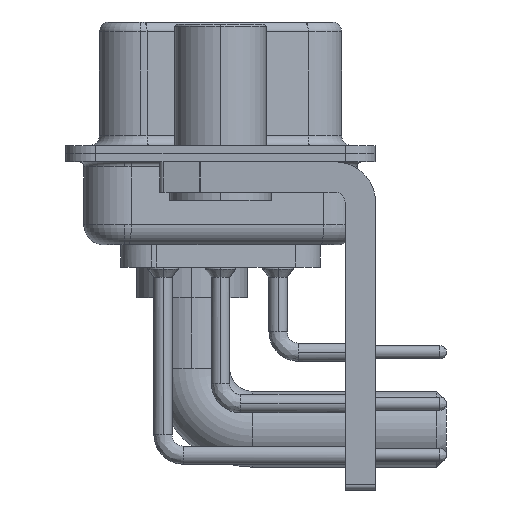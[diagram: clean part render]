
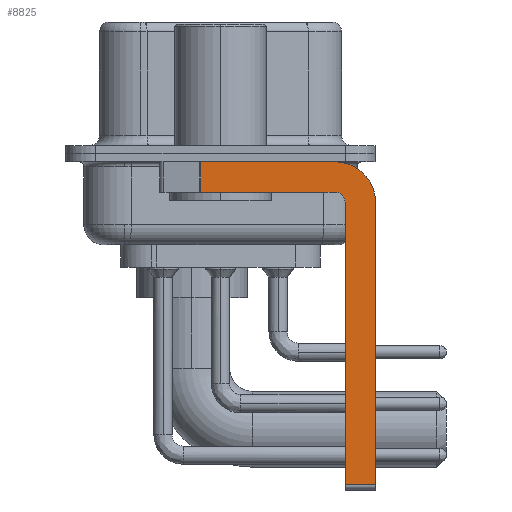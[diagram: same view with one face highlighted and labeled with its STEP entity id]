
A CAD part, left-side view. The second image highlights one B-rep face of the part: STEP entity #8825.
In plain terms, the highlighted planar face has unit normal (-1, 0, 0).
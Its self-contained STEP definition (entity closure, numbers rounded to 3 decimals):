
#295 = EDGE_LOOP ( 'NONE', ( #24912, #34311, #26086, #13538, #4832, #24836, #29060, #19026 ) ) ;
#925 = EDGE_CURVE ( 'NONE', #3163, #36008, #24729, .T. ) ;
#1463 = LINE ( 'NONE', #37172, #24164 ) ;
#2864 = VERTEX_POINT ( 'NONE', #9417 ) ;
#3163 = VERTEX_POINT ( 'NONE', #17668 ) ;
#3629 = CARTESIAN_POINT ( 'NONE',  ( -2.9, -5.65, -2.4 ) ) ;
#4257 = CIRCLE ( 'NONE', #36203, 2. ) ;
#4462 = VERTEX_POINT ( 'NONE', #5846 ) ;
#4832 = ORIENTED_EDGE ( 'NONE', *, *, #34094, .F. ) ;
#5170 = CARTESIAN_POINT ( 'NONE',  ( -2.9, -5.65, -2.4 ) ) ;
#5846 = CARTESIAN_POINT ( 'NONE',  ( -2.9, -5.65, -1.9 ) ) ;
#6271 = CARTESIAN_POINT ( 'NONE',  ( -2.9, -6.15, -16.6 ) ) ;
#6562 = DIRECTION ( 'NONE',  ( 0., -1., 0. ) ) ;
#7329 = EDGE_CURVE ( 'NONE', #3163, #32283, #21531, .T. ) ;
#7359 = DIRECTION ( 'NONE',  ( 0., 0., -1. ) ) ;
#7927 = DIRECTION ( 'NONE',  ( 0., 0., -1. ) ) ;
#8450 = DIRECTION ( 'NONE',  ( 0., -1., 0. ) ) ;
#8825 = ADVANCED_FACE ( 'NONE', ( #11072 ), #37724, .F. ) ;
#9406 = VECTOR ( 'NONE', #8450, 1000. ) ;
#9417 = CARTESIAN_POINT ( 'NONE',  ( -2.9, -7.65, -16.35 ) ) ;
#9419 = DIRECTION ( 'NONE',  ( 0., 0., 1. ) ) ;
#10335 = EDGE_CURVE ( 'NONE', #34247, #2864, #17264, .T. ) ;
#11072 = FACE_OUTER_BOUND ( 'NONE', #295, .T. ) ;
#12966 = CARTESIAN_POINT ( 'NONE',  ( -2.9, -7.65, -2.4 ) ) ;
#13329 = VECTOR ( 'NONE', #36632, 1000. ) ;
#13538 = ORIENTED_EDGE ( 'NONE', *, *, #33758, .F. ) ;
#13599 = DIRECTION ( 'NONE',  ( -1., 0., 0. ) ) ;
#13744 = VERTEX_POINT ( 'NONE', #27422 ) ;
#13748 = EDGE_CURVE ( 'NONE', #32283, #34247, #4257, .T. ) ;
#13773 = CARTESIAN_POINT ( 'NONE',  ( -2.9, -5.65, -16.35 ) ) ;
#14058 = AXIS2_PLACEMENT_3D ( 'NONE', #5170, #32456, #7927 ) ;
#14099 = CARTESIAN_POINT ( 'NONE',  ( -2.9, -7.65, -2.4 ) ) ;
#17264 = LINE ( 'NONE', #14099, #32358 ) ;
#17324 = LINE ( 'NONE', #13773, #9406 ) ;
#17668 = CARTESIAN_POINT ( 'NONE',  ( -2.9, 0.978, -0.4 ) ) ;
#19026 = ORIENTED_EDGE ( 'NONE', *, *, #13748, .F. ) ;
#19374 = DIRECTION ( 'NONE',  ( 0., 1., 0. ) ) ;
#21531 = LINE ( 'NONE', #33454, #24898 ) ;
#22760 = DIRECTION ( 'NONE',  ( 0., 0., -1. ) ) ;
#24164 = VECTOR ( 'NONE', #19374, 1000. ) ;
#24376 = LINE ( 'NONE', #6271, #35639 ) ;
#24729 = LINE ( 'NONE', #36246, #13329 ) ;
#24836 = ORIENTED_EDGE ( 'NONE', *, *, #36698, .T. ) ;
#24898 = VECTOR ( 'NONE', #6562, 1000. ) ;
#24912 = ORIENTED_EDGE ( 'NONE', *, *, #7329, .F. ) ;
#25575 = DIRECTION ( 'NONE',  ( 0., 0., 1. ) ) ;
#26086 = ORIENTED_EDGE ( 'NONE', *, *, #32454, .F. ) ;
#27422 = CARTESIAN_POINT ( 'NONE',  ( -2.9, -6.15, -2.4 ) ) ;
#27506 = CIRCLE ( 'NONE', #34999, 0.5 ) ;
#28375 = CARTESIAN_POINT ( 'NONE',  ( -2.9, 0.978, -1.9 ) ) ;
#28525 = CARTESIAN_POINT ( 'NONE',  ( -2.9, -5.65, -0.4 ) ) ;
#29060 = ORIENTED_EDGE ( 'NONE', *, *, #10335, .F. ) ;
#29485 = VERTEX_POINT ( 'NONE', #35802 ) ;
#32283 = VERTEX_POINT ( 'NONE', #28525 ) ;
#32358 = VECTOR ( 'NONE', #22760, 1000. ) ;
#32454 = EDGE_CURVE ( 'NONE', #4462, #36008, #1463, .T. ) ;
#32456 = DIRECTION ( 'NONE',  ( 1., 0., 0. ) ) ;
#33454 = CARTESIAN_POINT ( 'NONE',  ( -2.9, 3., -0.4 ) ) ;
#33758 = EDGE_CURVE ( 'NONE', #13744, #4462, #27506, .T. ) ;
#33989 = CARTESIAN_POINT ( 'NONE',  ( -2.9, -5.65, -2.4 ) ) ;
#34094 = EDGE_CURVE ( 'NONE', #29485, #13744, #24376, .T. ) ;
#34247 = VERTEX_POINT ( 'NONE', #12966 ) ;
#34311 = ORIENTED_EDGE ( 'NONE', *, *, #925, .T. ) ;
#34999 = AXIS2_PLACEMENT_3D ( 'NONE', #33989, #13599, #25575 ) ;
#35639 = VECTOR ( 'NONE', #9419, 1000. ) ;
#35802 = CARTESIAN_POINT ( 'NONE',  ( -2.9, -6.15, -16.35 ) ) ;
#36008 = VERTEX_POINT ( 'NONE', #28375 ) ;
#36203 = AXIS2_PLACEMENT_3D ( 'NONE', #3629, #36401, #7359 ) ;
#36246 = CARTESIAN_POINT ( 'NONE',  ( -2.9, 0.978, -1.9 ) ) ;
#36401 = DIRECTION ( 'NONE',  ( 1., 0., 0. ) ) ;
#36632 = DIRECTION ( 'NONE',  ( 0., 0., -1. ) ) ;
#36698 = EDGE_CURVE ( 'NONE', #29485, #2864, #17324, .T. ) ;
#37172 = CARTESIAN_POINT ( 'NONE',  ( -2.9, -5.65, -1.9 ) ) ;
#37724 = PLANE ( 'NONE',  #14058 ) ;
